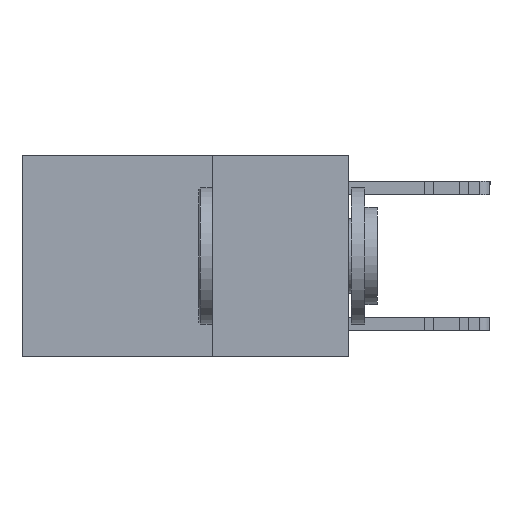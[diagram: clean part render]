
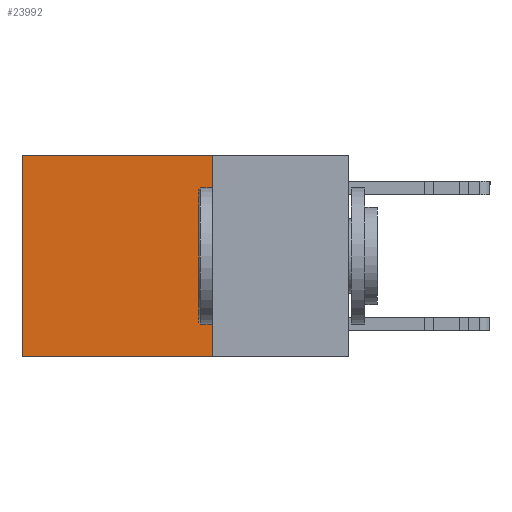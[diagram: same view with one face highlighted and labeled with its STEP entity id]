
A CAD part, left-side view. The second image highlights one B-rep face of the part: STEP entity #23992.
In plain terms, the highlighted planar face has unit normal (-1, 0, 0).
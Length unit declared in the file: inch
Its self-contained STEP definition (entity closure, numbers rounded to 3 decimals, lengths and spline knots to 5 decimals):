
#3083 = VECTOR ( 'NONE', #11142, 39.37008 ) ;
#3260 = VERTEX_POINT ( 'NONE', #11424 ) ;
#3564 = CARTESIAN_POINT ( 'NONE',  ( 0.2625, 0.25, 0. ) ) ;
#3567 = VERTEX_POINT ( 'NONE', #3564 ) ;
#3727 = LINE ( 'NONE', #31110, #25779 ) ;
#4079 = EDGE_CURVE ( 'NONE', #3567, #9637, #18799, .T. ) ;
#4259 = DIRECTION ( 'NONE',  ( 0., 0., -1. ) ) ;
#4414 = LINE ( 'NONE', #24929, #7482 ) ;
#5651 = CARTESIAN_POINT ( 'NONE',  ( 0.2625, 0.6, -0.37 ) ) ;
#7482 = VECTOR ( 'NONE', #14334, 39.37008 ) ;
#8246 = ORIENTED_EDGE ( 'NONE', *, *, #30686, .F. ) ;
#8658 = AXIS2_PLACEMENT_3D ( 'NONE', #11740, #21882, #4259 ) ;
#9452 = PLANE ( 'NONE',  #8658 ) ;
#9637 = VERTEX_POINT ( 'NONE', #30413 ) ;
#10791 = EDGE_CURVE ( 'NONE', #3260, #11606, #4414, .T. ) ;
#11142 = DIRECTION ( 'NONE',  ( 0., 0., -1. ) ) ;
#11424 = CARTESIAN_POINT ( 'NONE',  ( 0.2625, 0.6, 0. ) ) ;
#11467 = EDGE_LOOP ( 'NONE', ( #15065, #8246, #30610, #26817 ) ) ;
#11606 = VERTEX_POINT ( 'NONE', #5651 ) ;
#11740 = CARTESIAN_POINT ( 'NONE',  ( 0.2625, 0.25, 0. ) ) ;
#13630 = DIRECTION ( 'NONE',  ( 0., 1., 0. ) ) ;
#14334 = DIRECTION ( 'NONE',  ( 0., 0., -1. ) ) ;
#15065 = ORIENTED_EDGE ( 'NONE', *, *, #10791, .T. ) ;
#18198 = CARTESIAN_POINT ( 'NONE',  ( 0.2625, 0.25, -0.37 ) ) ;
#18478 = CARTESIAN_POINT ( 'NONE',  ( 0.2625, 0.25, 0. ) ) ;
#18799 = LINE ( 'NONE', #18478, #3083 ) ;
#18897 = FACE_OUTER_BOUND ( 'NONE', #11467, .T. ) ;
#21882 = DIRECTION ( 'NONE',  ( 1., 0., 0. ) ) ;
#21884 = EDGE_CURVE ( 'NONE', #3567, #3260, #3727, .T. ) ;
#23992 = ADVANCED_FACE ( 'NONE', ( #18897 ), #9452, .F. ) ;
#24929 = CARTESIAN_POINT ( 'NONE',  ( 0.2625, 0.6, 0. ) ) ;
#25779 = VECTOR ( 'NONE', #13630, 39.37008 ) ;
#26076 = LINE ( 'NONE', #18198, #28223 ) ;
#26817 = ORIENTED_EDGE ( 'NONE', *, *, #21884, .T. ) ;
#28223 = VECTOR ( 'NONE', #28345, 39.37008 ) ;
#28345 = DIRECTION ( 'NONE',  ( 0., 1., 0. ) ) ;
#30413 = CARTESIAN_POINT ( 'NONE',  ( 0.2625, 0.25, -0.37 ) ) ;
#30610 = ORIENTED_EDGE ( 'NONE', *, *, #4079, .F. ) ;
#30686 = EDGE_CURVE ( 'NONE', #9637, #11606, #26076, .T. ) ;
#31110 = CARTESIAN_POINT ( 'NONE',  ( 0.2625, 0.25, 0. ) ) ;
